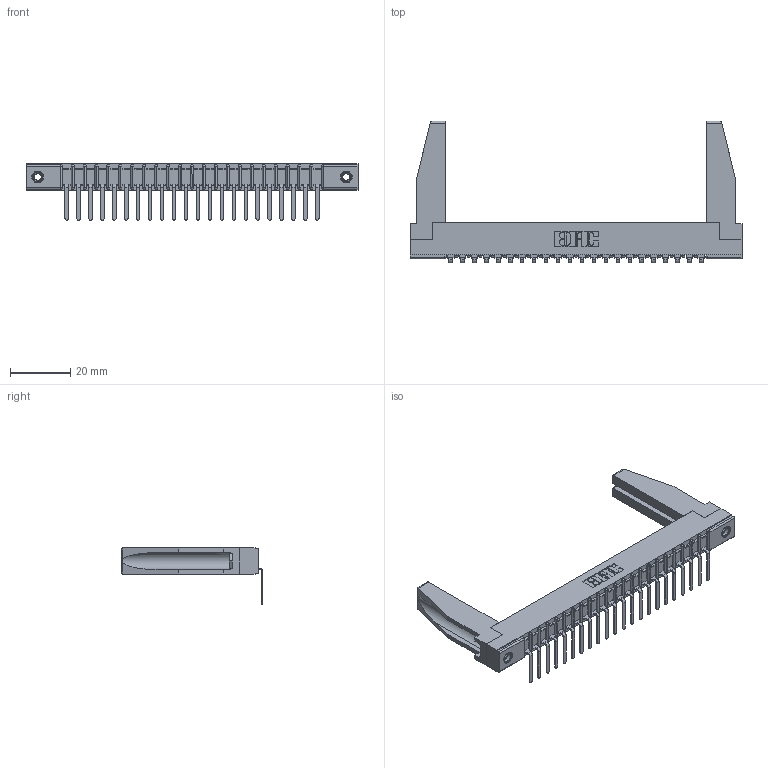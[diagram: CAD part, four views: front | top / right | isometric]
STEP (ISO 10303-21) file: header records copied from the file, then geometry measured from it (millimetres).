
FILE_DESCRIPTION (( 'STEP AP203' ), '1' );
FILE_NAME ('307-022-457-178.STEP', '2020-09-27T07:27:24', ( '' ), ( '' ), 'SwSTEP 2.0', 'SolidWorks 2020', '' );
FILE_SCHEMA (( 'CONFIG_CONTROL_DESIGN' ));
Length unit declared in the file: inch
Products named in the file (5): 345-250-001_345-250-001-102; 307-022-457-178; 307-220-078; 307-290-002_557; 307 Part_.156 Dia Mounting Holes
Assembly tree (27 placements, depth 2):
  307-022-457-178
    307 Part_.156 Dia Mounting Holes
    307-290-002_557  x22
    307-220-078  x2
    345-250-001_345-250-001-102  x2
Bounding box: 110.19 x 47.03 x 18.67 mm (x, y, z)
Volume: 11326.9 mm3; surface area: 17522.1 mm2
Topology: 27 solids, 27 shells, 1987 faces, 6021 edges, 3942 vertices
Faces by surface type: plane 1188, cylinder 737, sphere 46, cone 12, torus 4
Entity records: 24619 total; most frequent: CARTESIAN_POINT 4150, ORIENTED_EDGE 4096, DIRECTION 3998, EDGE_CURVE 2048, VECTOR 1562, LINE 1562, VERTEX_POINT 1328, AXIS2_PLACEMENT_3D 1218
